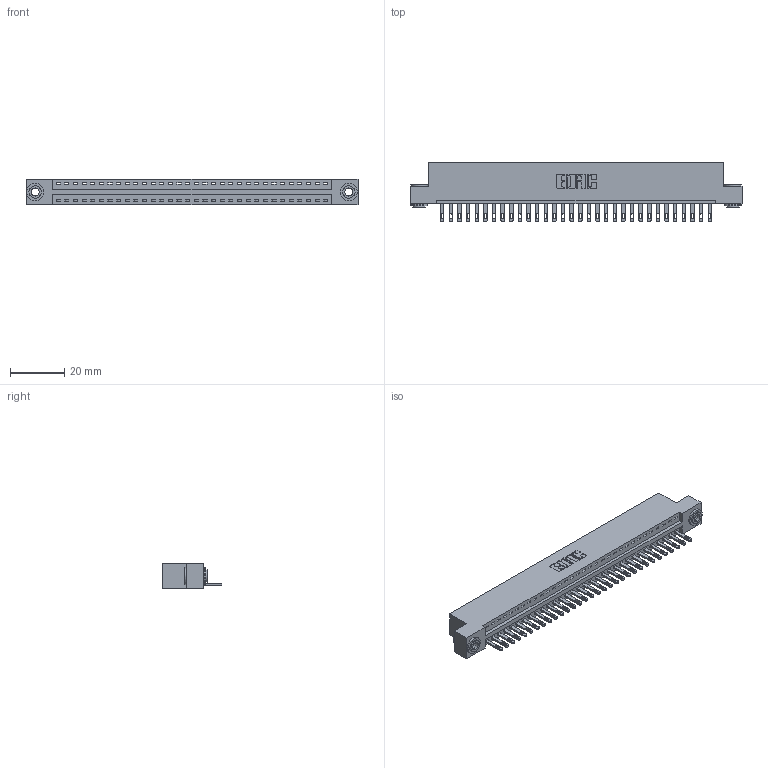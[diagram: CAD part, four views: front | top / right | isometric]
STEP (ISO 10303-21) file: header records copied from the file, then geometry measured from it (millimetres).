
FILE_DESCRIPTION (( 'STEP AP203' ), '1' );
FILE_NAME ('346-032-500-103.STEP', '2022-05-06T17:40:21', ( '' ), ( '' ), 'SwSTEP 2.0', 'SolidWorks 2020', '' );
FILE_SCHEMA (( 'CONFIG_CONTROL_DESIGN' ));
Length unit declared in the file: inch
Products named in the file (4): 346 Part_Flush Mounting Lugs - 0.156 Dia-TH; 345-250-002_345-250-002-102; 345-292-001_345-293-100; 346-032-500-103
Assembly tree (35 placements, depth 2):
  346-032-500-103
    346 Part_Flush Mounting Lugs - 0.156 Dia-TH
    345-292-001_345-293-100  x32
    345-250-002_345-250-002-102  x2
Bounding box: 122.17 x 21.84 x 9.4 mm (x, y, z)
Volume: 11647 mm3; surface area: 14775.3 mm2
Topology: 35 solids, 35 shells, 1902 faces, 5817 edges, 3874 vertices
Faces by surface type: plane 1188, cylinder 706, cone 8
Entity records: 22202 total; most frequent: CARTESIAN_POINT 3789, ORIENTED_EDGE 3746, DIRECTION 3387, EDGE_CURVE 1873, LINE 1585, VECTOR 1585, VERTEX_POINT 1246, AXIS2_PLACEMENT_3D 901
